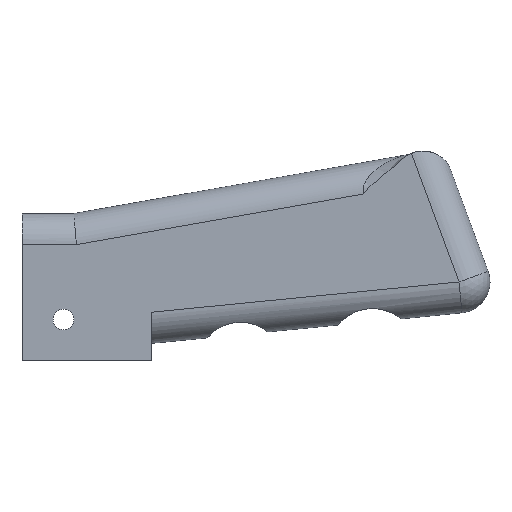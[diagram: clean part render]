
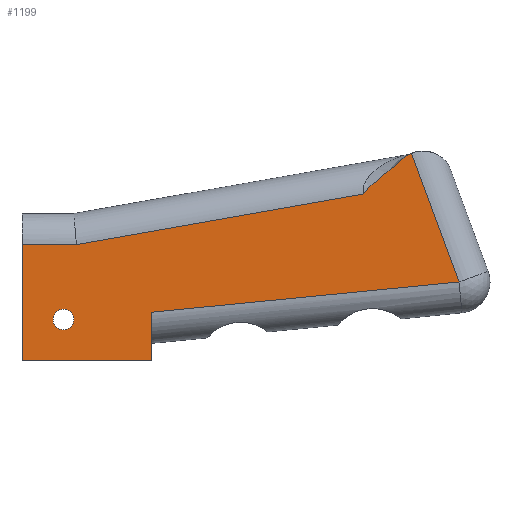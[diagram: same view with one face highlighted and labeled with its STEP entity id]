
A CAD part, left-side view. The second image highlights one B-rep face of the part: STEP entity #1199.
In plain terms, the highlighted planar face has unit normal (-1, 0, 0).
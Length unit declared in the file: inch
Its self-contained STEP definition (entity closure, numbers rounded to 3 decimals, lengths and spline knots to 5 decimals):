
#9 = EDGE_CURVE ( 'NONE', #1437, #768, #374, .T. ) ;
#11 = CARTESIAN_POINT ( 'NONE',  ( -0.4375, -2.07017, 0.98702 ) ) ;
#12 = DIRECTION ( 'NONE',  ( 0., -0.995, 0.098 ) ) ;
#21 = CARTESIAN_POINT ( 'NONE',  ( -0.4375, -2.20248, 1.11712 ) ) ;
#27 = VERTEX_POINT ( 'NONE', #834 ) ;
#63 = VERTEX_POINT ( 'NONE', #1080 ) ;
#64 = CARTESIAN_POINT ( 'NONE',  ( -0.4375, 0., -0.17856 ) ) ;
#72 = ORIENTED_EDGE ( 'NONE', *, *, #1729, .F. ) ;
#85 = DIRECTION ( 'NONE',  ( 1., 0., 0. ) ) ;
#140 = FACE_OUTER_BOUND ( 'NONE', #1685, .T. ) ;
#141 = ORIENTED_EDGE ( 'NONE', *, *, #1581, .T. ) ;
#143 = CARTESIAN_POINT ( 'NONE',  ( -0.4375, 0., 0.65 ) ) ;
#209 = EDGE_CURVE ( 'NONE', #63, #1623, #528, .T. ) ;
#266 = B_SPLINE_CURVE_WITH_KNOTS ( 'NONE', 3,
 ( #566, #1686, #433, #21, #297, #573, #843, #993, #286, #11, #1142, #1136, #849, #836 ),
 .UNSPECIFIED., .F., .F.,
 ( 4, 2, 2, 2, 2, 2, 4 ),
 ( 0., 0.00646, 0.00968, 0.0113, 0.01211, 0.01251, 0.01291 ),
 .UNSPECIFIED. ) ;
#280 = VERTEX_POINT ( 'NONE', #1714 ) ;
#286 = CARTESIAN_POINT ( 'NONE',  ( -0.4375, -2.07982, 0.99985 ) ) ;
#296 = ORIENTED_EDGE ( 'NONE', *, *, #666, .T. ) ;
#297 = CARTESIAN_POINT ( 'NONE',  ( -0.4375, -2.16928, 1.09078 ) ) ;
#300 = VERTEX_POINT ( 'NONE', #415 ) ;
#313 = VERTEX_POINT ( 'NONE', #470 ) ;
#349 = VECTOR ( 'NONE', #396, 39.37008 ) ;
#374 = LINE ( 'NONE', #393, #705 ) ;
#393 = CARTESIAN_POINT ( 'NONE',  ( -0.4375, 0.69791, 0.47956 ) ) ;
#396 = DIRECTION ( 'NONE',  ( 0., -1., 0. ) ) ;
#415 = CARTESIAN_POINT ( 'NONE',  ( -0.4375, 0., -0.65 ) ) ;
#433 = CARTESIAN_POINT ( 'NONE',  ( -0.4375, -2.30291, 1.19517 ) ) ;
#465 = LINE ( 'NONE', #972, #959 ) ;
#470 = CARTESIAN_POINT ( 'NONE',  ( -0.4375, -2.43348, 1.3032 ) ) ;
#500 = CARTESIAN_POINT ( 'NONE',  ( -0.4375, 0., 0.65 ) ) ;
#528 = LINE ( 'NONE', #1531, #1249 ) ;
#565 = CARTESIAN_POINT ( 'NONE',  ( -0.4375, 0.85, -0.25 ) ) ;
#566 = CARTESIAN_POINT ( 'NONE',  ( -0.4375, -2.43348, 1.3032 ) ) ;
#569 = EDGE_CURVE ( 'NONE', #1628, #1672, #1703, .T. ) ;
#573 = CARTESIAN_POINT ( 'NONE',  ( -0.4375, -2.12265, 1.0475 ) ) ;
#591 = ORIENTED_EDGE ( 'NONE', *, *, #9, .T. ) ;
#592 = CARTESIAN_POINT ( 'NONE',  ( -0.4375, 1.25, 0.65 ) ) ;
#603 = ORIENTED_EDGE ( 'NONE', *, *, #209, .T. ) ;
#618 = EDGE_CURVE ( 'NONE', #877, #63, #1274, .T. ) ;
#635 = ORIENTED_EDGE ( 'NONE', *, *, #1397, .T. ) ;
#637 = CARTESIAN_POINT ( 'NONE',  ( -0.4375, 0.72376, 0.475 ) ) ;
#640 = ORIENTED_EDGE ( 'NONE', *, *, #618, .T. ) ;
#645 = DIRECTION ( 'NONE',  ( 0., 0., -1. ) ) ;
#662 = ORIENTED_EDGE ( 'NONE', *, *, #1439, .T. ) ;
#666 = EDGE_CURVE ( 'NONE', #768, #280, #465, .T. ) ;
#701 = CARTESIAN_POINT ( 'NONE',  ( -0.4375, -2.51593, 1.35669 ) ) ;
#705 = VECTOR ( 'NONE', #792, 39.37008 ) ;
#716 = CARTESIAN_POINT ( 'NONE',  ( -0.4375, -2.05509, 0.9649 ) ) ;
#723 = DIRECTION ( 'NONE',  ( 0., 0., 1. ) ) ;
#768 = VERTEX_POINT ( 'NONE', #637 ) ;
#783 = PLANE ( 'NONE',  #1132 ) ;
#792 = DIRECTION ( 'NONE',  ( 0., 0.985, -0.174 ) ) ;
#834 = CARTESIAN_POINT ( 'NONE',  ( -0.4375, 1.25, -0.65 ) ) ;
#836 = CARTESIAN_POINT ( 'NONE',  ( -0.4375, -2.05509, 0.9649 ) ) ;
#843 = CARTESIAN_POINT ( 'NONE',  ( -0.4375, -2.10765, 1.03241 ) ) ;
#849 = CARTESIAN_POINT ( 'NONE',  ( -0.4375, -2.05794, 0.96937 ) ) ;
#862 = CARTESIAN_POINT ( 'NONE',  ( -0.4375, 0.85, -0.35 ) ) ;
#877 = VERTEX_POINT ( 'NONE', #64 ) ;
#921 = ORIENTED_EDGE ( 'NONE', *, *, #1169, .T. ) ;
#943 = DIRECTION ( 'NONE',  ( 0., 0., 1. ) ) ;
#959 = VECTOR ( 'NONE', #1687, 39.37008 ) ;
#968 = CARTESIAN_POINT ( 'NONE',  ( -0.4375, 0., -0.65 ) ) ;
#971 = CIRCLE ( 'NONE', #1086, 0.1 ) ;
#972 = CARTESIAN_POINT ( 'NONE',  ( -0.4375, 1.25, 0.475 ) ) ;
#979 = CARTESIAN_POINT ( 'NONE',  ( -0.4375, -2.62911, 1.09196 ) ) ;
#993 = CARTESIAN_POINT ( 'NONE',  ( -0.4375, -2.08657, 1.00815 ) ) ;
#1043 = CIRCLE ( 'NONE', #1515, 0.28791 ) ;
#1080 = CARTESIAN_POINT ( 'NONE',  ( -0.4375, -2.97536, 0.11351 ) ) ;
#1086 = AXIS2_PLACEMENT_3D ( 'NONE', #565, #1417, #1549 ) ;
#1121 = ORIENTED_EDGE ( 'NONE', *, *, #569, .F. ) ;
#1126 = DIRECTION ( 'NONE',  ( 0., 0., -1. ) ) ;
#1131 = LINE ( 'NONE', #968, #349 ) ;
#1132 = AXIS2_PLACEMENT_3D ( 'NONE', #500, #85, #645 ) ;
#1136 = CARTESIAN_POINT ( 'NONE',  ( -0.4375, -2.06093, 0.97388 ) ) ;
#1142 = CARTESIAN_POINT ( 'NONE',  ( -0.4375, -2.06704, 0.98268 ) ) ;
#1169 = EDGE_CURVE ( 'NONE', #280, #27, #1213, .T. ) ;
#1199 = ADVANCED_FACE ( 'NONE', ( #1311, #140 ), #783, .F. ) ;
#1213 = LINE ( 'NONE', #592, #1461 ) ;
#1217 = DIRECTION ( 'NONE',  ( 0., 0., -1. ) ) ;
#1235 = CARTESIAN_POINT ( 'NONE',  ( -0.4375, -0.51445, -0.12806 ) ) ;
#1249 = VECTOR ( 'NONE', #1671, 39.37008 ) ;
#1274 = LINE ( 'NONE', #1235, #1596 ) ;
#1307 = LINE ( 'NONE', #143, #1352 ) ;
#1311 = FACE_BOUND ( 'NONE', #1431, .T. ) ;
#1352 = VECTOR ( 'NONE', #1126, 39.37008 ) ;
#1382 = AXIS2_PLACEMENT_3D ( 'NONE', #1766, #1610, #943 ) ;
#1397 = EDGE_CURVE ( 'NONE', #313, #1437, #266, .T. ) ;
#1417 = DIRECTION ( 'NONE',  ( -1., 0., 0. ) ) ;
#1431 = EDGE_LOOP ( 'NONE', ( #1520, #1121 ) ) ;
#1437 = VERTEX_POINT ( 'NONE', #716 ) ;
#1439 = EDGE_CURVE ( 'NONE', #1623, #313, #1043, .T. ) ;
#1461 = VECTOR ( 'NONE', #1217, 39.37008 ) ;
#1515 = AXIS2_PLACEMENT_3D ( 'NONE', #979, #1556, #723 ) ;
#1520 = ORIENTED_EDGE ( 'NONE', *, *, #1667, .F. ) ;
#1531 = CARTESIAN_POINT ( 'NONE',  ( -0.4375, -2.60302, 1.12105 ) ) ;
#1549 = DIRECTION ( 'NONE',  ( 0., 0., 1. ) ) ;
#1556 = DIRECTION ( 'NONE',  ( -1., 0., 0. ) ) ;
#1581 = EDGE_CURVE ( 'NONE', #27, #300, #1131, .T. ) ;
#1596 = VECTOR ( 'NONE', #12, 39.37008 ) ;
#1610 = DIRECTION ( 'NONE',  ( -1., 0., 0. ) ) ;
#1623 = VERTEX_POINT ( 'NONE', #701 ) ;
#1628 = VERTEX_POINT ( 'NONE', #862 ) ;
#1667 = EDGE_CURVE ( 'NONE', #1672, #1628, #971, .T. ) ;
#1671 = DIRECTION ( 'NONE',  ( 0., 0.347, 0.938 ) ) ;
#1672 = VERTEX_POINT ( 'NONE', #1698 ) ;
#1685 = EDGE_LOOP ( 'NONE', ( #640, #603, #662, #635, #591, #296, #921, #141, #72 ) ) ;
#1686 = CARTESIAN_POINT ( 'NONE',  ( -0.4375, -2.37125, 1.24556 ) ) ;
#1687 = DIRECTION ( 'NONE',  ( 0., 1., 0. ) ) ;
#1698 = CARTESIAN_POINT ( 'NONE',  ( -0.4375, 0.85, -0.15 ) ) ;
#1703 = CIRCLE ( 'NONE', #1382, 0.1 ) ;
#1714 = CARTESIAN_POINT ( 'NONE',  ( -0.4375, 1.25, 0.475 ) ) ;
#1729 = EDGE_CURVE ( 'NONE', #877, #300, #1307, .T. ) ;
#1766 = CARTESIAN_POINT ( 'NONE',  ( -0.4375, 0.85, -0.25 ) ) ;
